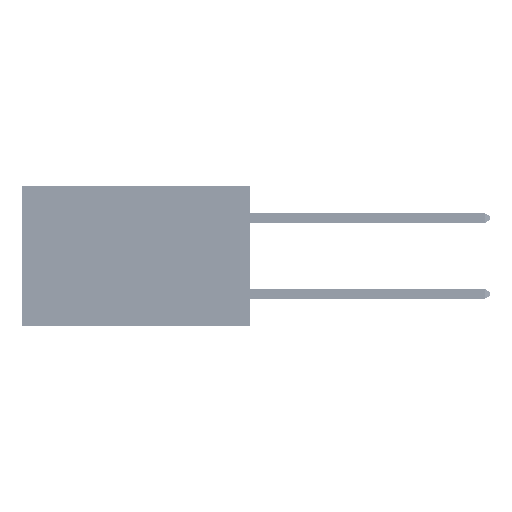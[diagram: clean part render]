
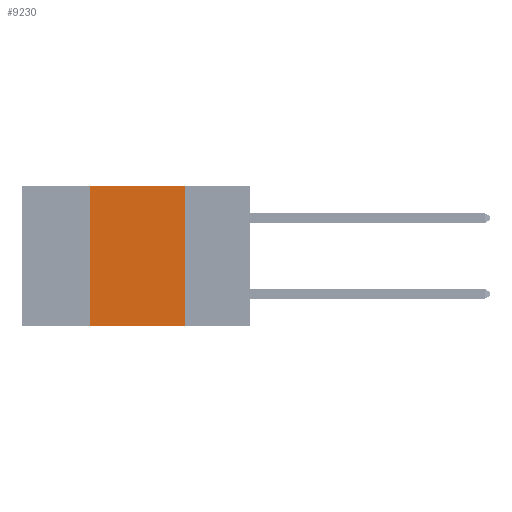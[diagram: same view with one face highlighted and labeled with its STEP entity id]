
A CAD part, left-side view. The second image highlights one B-rep face of the part: STEP entity #9230.
In plain terms, the highlighted planar face has unit normal (-1, 0, 0).
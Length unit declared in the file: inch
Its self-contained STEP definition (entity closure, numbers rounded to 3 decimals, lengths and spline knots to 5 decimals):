
#1279 = LINE ( 'NONE', #33145, #25880 ) ;
#1377 = VERTEX_POINT ( 'NONE', #32975 ) ;
#1440 = FACE_OUTER_BOUND ( 'NONE', #31478, .T. ) ;
#3861 = EDGE_CURVE ( 'NONE', #40580, #8546, #25629, .T. ) ;
#6012 = CARTESIAN_POINT ( 'NONE',  ( 0., 0.42, -0.37 ) ) ;
#6330 = ORIENTED_EDGE ( 'NONE', *, *, #22827, .F. ) ;
#6826 = DIRECTION ( 'NONE',  ( 0., 0., 1. ) ) ;
#6852 = DIRECTION ( 'NONE',  ( 0., -1., 0. ) ) ;
#7408 = DIRECTION ( 'NONE',  ( 0., 0., -1. ) ) ;
#8041 = PLANE ( 'NONE',  #36727 ) ;
#8546 = VERTEX_POINT ( 'NONE', #33840 ) ;
#9230 = ADVANCED_FACE ( 'NONE', ( #1440 ), #8041, .F. ) ;
#9240 = ORIENTED_EDGE ( 'NONE', *, *, #36993, .F. ) ;
#9393 = VECTOR ( 'NONE', #6826, 39.37008 ) ;
#15384 = DIRECTION ( 'NONE',  ( 1., 0., 0. ) ) ;
#15758 = CARTESIAN_POINT ( 'NONE',  ( 0., 0.42, 0. ) ) ;
#22827 = EDGE_CURVE ( 'NONE', #39101, #1377, #33003, .T. ) ;
#23756 = ORIENTED_EDGE ( 'NONE', *, *, #36267, .F. ) ;
#25629 = LINE ( 'NONE', #39606, #36543 ) ;
#25880 = VECTOR ( 'NONE', #7408, 39.37008 ) ;
#26067 = VECTOR ( 'NONE', #27237, 39.37008 ) ;
#26396 = DIRECTION ( 'NONE',  ( 0., 0., -1. ) ) ;
#27237 = DIRECTION ( 'NONE',  ( 0., -1., 0. ) ) ;
#31264 = CARTESIAN_POINT ( 'NONE',  ( 0., 0.6, 0. ) ) ;
#31478 = EDGE_LOOP ( 'NONE', ( #9240, #6330, #23756, #45258 ) ) ;
#31684 = LINE ( 'NONE', #43295, #9393 ) ;
#32975 = CARTESIAN_POINT ( 'NONE',  ( 0., 0.17, 0. ) ) ;
#33003 = LINE ( 'NONE', #31264, #26067 ) ;
#33145 = CARTESIAN_POINT ( 'NONE',  ( 0., 0.17, 0. ) ) ;
#33640 = CARTESIAN_POINT ( 'NONE',  ( 0., 0.6, 0. ) ) ;
#33840 = CARTESIAN_POINT ( 'NONE',  ( 0., 0.17, -0.37 ) ) ;
#36267 = EDGE_CURVE ( 'NONE', #40580, #39101, #31684, .T. ) ;
#36543 = VECTOR ( 'NONE', #6852, 39.37008 ) ;
#36727 = AXIS2_PLACEMENT_3D ( 'NONE', #33640, #15384, #26396 ) ;
#36993 = EDGE_CURVE ( 'NONE', #1377, #8546, #1279, .T. ) ;
#39101 = VERTEX_POINT ( 'NONE', #15758 ) ;
#39606 = CARTESIAN_POINT ( 'NONE',  ( 0., 0.6, -0.37 ) ) ;
#40580 = VERTEX_POINT ( 'NONE', #6012 ) ;
#43295 = CARTESIAN_POINT ( 'NONE',  ( 0., 0.42, 0. ) ) ;
#45258 = ORIENTED_EDGE ( 'NONE', *, *, #3861, .T. ) ;
